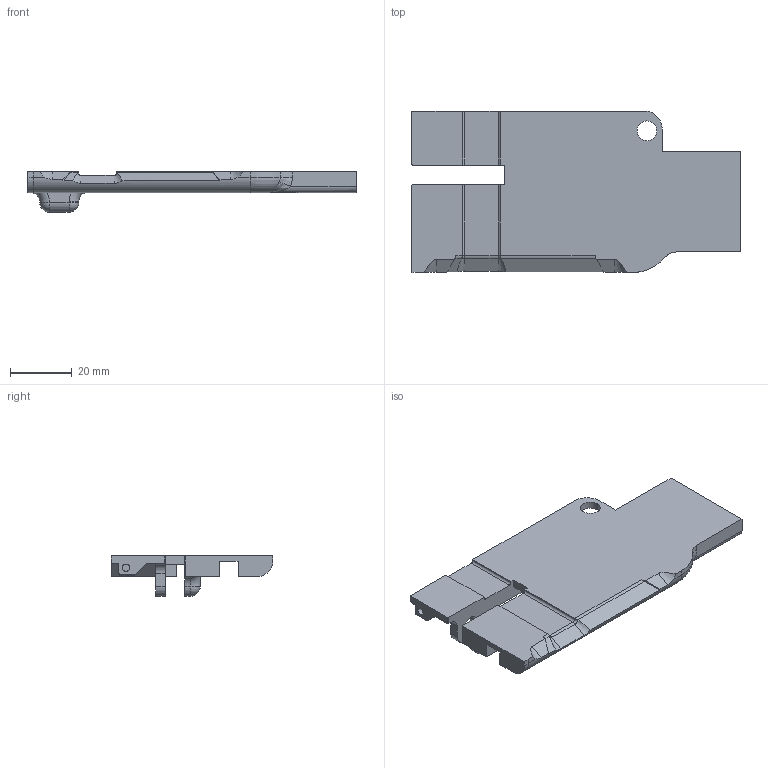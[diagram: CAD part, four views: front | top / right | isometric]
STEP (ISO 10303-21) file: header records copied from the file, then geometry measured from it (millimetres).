
FILE_DESCRIPTION (( 'STEP AP214' ), '1' );
FILE_NAME ('Receiver_Magwell_Left.step', '2014-05-14T06:10:03', ( 'WarFairy' ), ( '' ), 'SwSTEP 2.0', 'SolidWorks 2013', '' );
FILE_SCHEMA (( 'AUTOMOTIVE_DESIGN' ));
Length unit declared in the file: inch
Products named in the file (1): Receiver_Magwell_Left
Bounding box: 106.45 x 52.34 x 13.07 mm (x, y, z)
Volume: 24673.6 mm3; surface area: 13823.6 mm2
Topology: 1 solids, 1 shells, 128 faces, 344 edges, 214 vertices
Faces by surface type: plane 63, cylinder 47, torus 7, cone 4, sphere 4, bspline 3
Entity records: 4260 total; most frequent: CARTESIAN_POINT 1023, ORIENTED_EDGE 680, DIRECTION 663, EDGE_CURVE 340, AXIS2_PLACEMENT_3D 222, VECTOR 219, LINE 219, VERTEX_POINT 214
